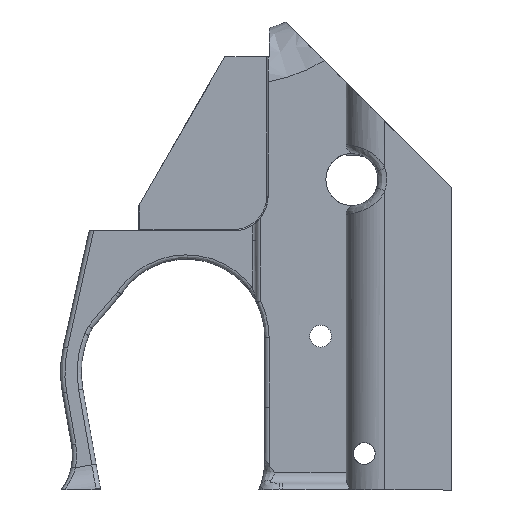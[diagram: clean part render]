
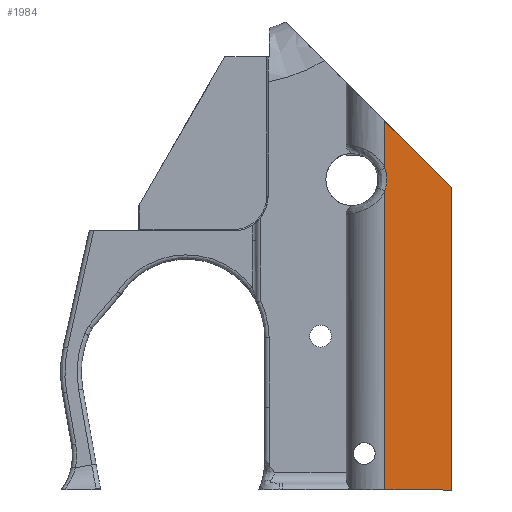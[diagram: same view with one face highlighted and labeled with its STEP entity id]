
A CAD part, front view. The second image highlights one B-rep face of the part: STEP entity #1984.
In plain terms, the highlighted planar face has unit normal (0, -1, 0).
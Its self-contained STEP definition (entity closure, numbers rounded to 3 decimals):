
#25 = ORIENTED_EDGE ( 'NONE', *, *, #2656, .T. ) ;
#568 = ORIENTED_EDGE ( 'NONE', *, *, #9132, .T. ) ;
#933 = VERTEX_POINT ( 'NONE', #16102 ) ;
#1209 = ORIENTED_EDGE ( 'NONE', *, *, #16597, .F. ) ;
#1977 = PLANE ( 'NONE',  #4998 ) ;
#1984 = ADVANCED_FACE ( 'NONE', ( #9215 ), #1977, .T. ) ;
#2056 = VECTOR ( 'NONE', #10454, 1000. ) ;
#2127 = LINE ( 'NONE', #7821, #2056 ) ;
#2653 = VERTEX_POINT ( 'NONE', #7991 ) ;
#2656 = EDGE_CURVE ( 'NONE', #16637, #13586, #8184, .T. ) ;
#2732 = VECTOR ( 'NONE', #12131, 1000. ) ;
#2822 = DIRECTION ( 'NONE',  ( -1., 0., 0. ) ) ;
#2986 = LINE ( 'NONE', #15801, #2732 ) ;
#3328 = CARTESIAN_POINT ( 'NONE',  ( 62.492, -57.955, -101.909 ) ) ;
#3500 = DIRECTION ( 'NONE',  ( 0., -1., 0. ) ) ;
#4053 = LINE ( 'NONE', #10632, #4235 ) ;
#4122 = CARTESIAN_POINT ( 'NONE',  ( 62.826, -57.955, 18.811 ) ) ;
#4235 = VECTOR ( 'NONE', #2822, 1000. ) ;
#4998 = AXIS2_PLACEMENT_3D ( 'NONE', #3328, #3500, #6634 ) ;
#5396 = CARTESIAN_POINT ( 'NONE',  ( 62.715, -57.955, 16.742 ) ) ;
#6300 = CARTESIAN_POINT ( 'NONE',  ( 74.612, -57.955, -123.414 ) ) ;
#6605 = CARTESIAN_POINT ( 'NONE',  ( 62.715, -57.955, 19.489 ) ) ;
#6634 = DIRECTION ( 'NONE',  ( 0., 0., -1. ) ) ;
#6709 = EDGE_CURVE ( 'NONE', #7557, #12327, #4053, .T. ) ;
#7051 = B_SPLINE_CURVE_WITH_KNOTS ( 'NONE', 3,
 ( #10587, #6605, #4122, #13143, #5396, #14414 ),
 .UNSPECIFIED., .F., .F.,
 ( 4, 2, 4 ),
 ( 0., 0.5, 1. ),
 .UNSPECIFIED. ) ;
#7123 = CARTESIAN_POINT ( 'NONE',  ( 127.833, -57.955, -36.568 ) ) ;
#7182 = DIRECTION ( 'NONE',  ( -0.707, 0., 0.707 ) ) ;
#7314 = CARTESIAN_POINT ( 'NONE',  ( 62.492, -57.955, 28.773 ) ) ;
#7557 = VERTEX_POINT ( 'NONE', #14504 ) ;
#7600 = DIRECTION ( 'NONE',  ( 0., 0., -1. ) ) ;
#7821 = CARTESIAN_POINT ( 'NONE',  ( 62.492, -57.955, -101.909 ) ) ;
#7991 = CARTESIAN_POINT ( 'NONE',  ( 62.492, -57.955, 20.148 ) ) ;
#8152 = VECTOR ( 'NONE', #7182, 1000. ) ;
#8184 = LINE ( 'NONE', #7123, #8152 ) ;
#8352 = ORIENTED_EDGE ( 'NONE', *, *, #6709, .F. ) ;
#8576 = EDGE_CURVE ( 'NONE', #933, #12327, #2127, .T. ) ;
#9132 = EDGE_CURVE ( 'NONE', #2653, #933, #7051, .T. ) ;
#9215 = FACE_OUTER_BOUND ( 'NONE', #13674, .T. ) ;
#9397 = ORIENTED_EDGE ( 'NONE', *, *, #8576, .T. ) ;
#9487 = ORIENTED_EDGE ( 'NONE', *, *, #14333, .T. ) ;
#10454 = DIRECTION ( 'NONE',  ( 0., 0., -1. ) ) ;
#10587 = CARTESIAN_POINT ( 'NONE',  ( 62.492, -57.955, 20.148 ) ) ;
#10632 = CARTESIAN_POINT ( 'NONE',  ( 62.492, -57.955, -38.511 ) ) ;
#12131 = DIRECTION ( 'NONE',  ( 0., 0., -1. ) ) ;
#12327 = VERTEX_POINT ( 'NONE', #14678 ) ;
#12859 = CARTESIAN_POINT ( 'NONE',  ( 74.612, -57.955, 16.653 ) ) ;
#13143 = CARTESIAN_POINT ( 'NONE',  ( 62.827, -57.955, 17.42 ) ) ;
#13586 = VERTEX_POINT ( 'NONE', #7314 ) ;
#13674 = EDGE_LOOP ( 'NONE', ( #1209, #25, #9487, #568, #9397, #8352 ) ) ;
#14333 = EDGE_CURVE ( 'NONE', #13586, #2653, #2986, .T. ) ;
#14414 = CARTESIAN_POINT ( 'NONE',  ( 62.492, -57.955, 16.082 ) ) ;
#14504 = CARTESIAN_POINT ( 'NONE',  ( 74.612, -57.955, -38.511 ) ) ;
#14678 = CARTESIAN_POINT ( 'NONE',  ( 62.492, -57.955, -38.511 ) ) ;
#15801 = CARTESIAN_POINT ( 'NONE',  ( 62.492, -57.955, -101.909 ) ) ;
#15982 = VECTOR ( 'NONE', #7600, 1000. ) ;
#16086 = LINE ( 'NONE', #6300, #15982 ) ;
#16102 = CARTESIAN_POINT ( 'NONE',  ( 62.492, -57.955, 16.082 ) ) ;
#16597 = EDGE_CURVE ( 'NONE', #16637, #7557, #16086, .T. ) ;
#16637 = VERTEX_POINT ( 'NONE', #12859 ) ;
